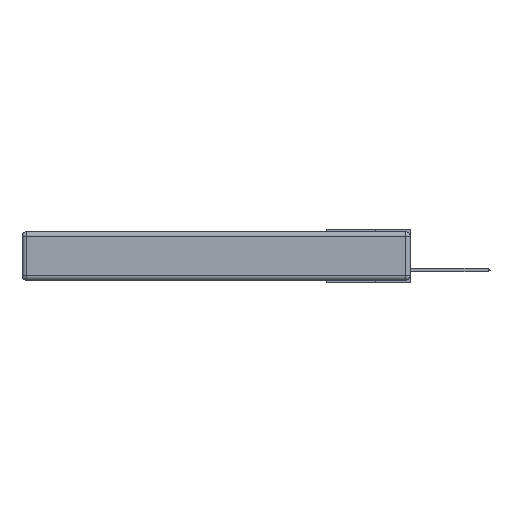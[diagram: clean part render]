
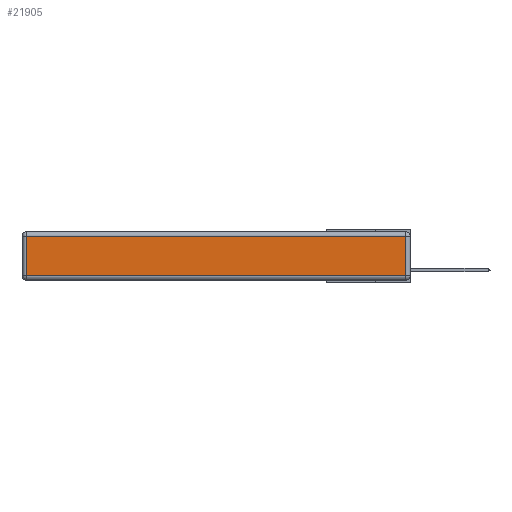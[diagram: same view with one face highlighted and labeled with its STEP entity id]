
A CAD part, left-side view. The second image highlights one B-rep face of the part: STEP entity #21905.
In plain terms, the highlighted planar face has unit normal (-1, 0, 0).
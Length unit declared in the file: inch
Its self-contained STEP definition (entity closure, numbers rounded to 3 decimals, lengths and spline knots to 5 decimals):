
#829 = VECTOR ( 'NONE', #23057, 39.37008 ) ;
#1310 = CARTESIAN_POINT ( 'NONE',  ( 0., 2.72, -0.343 ) ) ;
#1748 = ORIENTED_EDGE ( 'NONE', *, *, #15482, .T. ) ;
#3107 = CARTESIAN_POINT ( 'NONE',  ( 0., 2.72, -0.313 ) ) ;
#3405 = DIRECTION ( 'NONE',  ( 0., 0., 1. ) ) ;
#4110 = CARTESIAN_POINT ( 'NONE',  ( 0., 0., -0.343 ) ) ;
#4360 = FACE_OUTER_BOUND ( 'NONE', #23203, .T. ) ;
#4578 = CARTESIAN_POINT ( 'NONE',  ( 0., 2.72, -0.03 ) ) ;
#5504 = CARTESIAN_POINT ( 'NONE',  ( 0., 0.03, -0.03 ) ) ;
#5834 = LINE ( 'NONE', #1310, #16035 ) ;
#6849 = CARTESIAN_POINT ( 'NONE',  ( 0., 0.03, -0.313 ) ) ;
#7500 = ORIENTED_EDGE ( 'NONE', *, *, #12608, .T. ) ;
#8738 = ORIENTED_EDGE ( 'NONE', *, *, #14990, .T. ) ;
#12608 = EDGE_CURVE ( 'NONE', #20358, #20568, #19639, .T. ) ;
#13585 = VERTEX_POINT ( 'NONE', #4578 ) ;
#13968 = CARTESIAN_POINT ( 'NONE',  ( 0., 2.75, -0.03 ) ) ;
#14410 = AXIS2_PLACEMENT_3D ( 'NONE', #4110, #25110, #3405 ) ;
#14946 = ORIENTED_EDGE ( 'NONE', *, *, #26961, .T. ) ;
#14990 = EDGE_CURVE ( 'NONE', #20568, #25795, #22306, .T. ) ;
#15066 = DIRECTION ( 'NONE',  ( 0., 0., -1. ) ) ;
#15209 = DIRECTION ( 'NONE',  ( 0., -1., 0. ) ) ;
#15482 = EDGE_CURVE ( 'NONE', #25795, #13585, #22269, .T. ) ;
#16035 = VECTOR ( 'NONE', #15066, 39.37008 ) ;
#19605 = CARTESIAN_POINT ( 'NONE',  ( 0., 0., -0.313 ) ) ;
#19639 = LINE ( 'NONE', #19605, #27043 ) ;
#20358 = VERTEX_POINT ( 'NONE', #3107 ) ;
#20568 = VERTEX_POINT ( 'NONE', #6849 ) ;
#21048 = CARTESIAN_POINT ( 'NONE',  ( 0., 0.03, -0.343 ) ) ;
#21905 = ADVANCED_FACE ( 'NONE', ( #4360 ), #24318, .T. ) ;
#22269 = LINE ( 'NONE', #13968, #829 ) ;
#22306 = LINE ( 'NONE', #21048, #24755 ) ;
#23057 = DIRECTION ( 'NONE',  ( 0., 1., 0. ) ) ;
#23203 = EDGE_LOOP ( 'NONE', ( #7500, #8738, #1748, #14946 ) ) ;
#24318 = PLANE ( 'NONE',  #14410 ) ;
#24755 = VECTOR ( 'NONE', #27819, 39.37008 ) ;
#25110 = DIRECTION ( 'NONE',  ( -1., 0., 0. ) ) ;
#25795 = VERTEX_POINT ( 'NONE', #5504 ) ;
#26961 = EDGE_CURVE ( 'NONE', #13585, #20358, #5834, .T. ) ;
#27043 = VECTOR ( 'NONE', #15209, 39.37008 ) ;
#27819 = DIRECTION ( 'NONE',  ( 0., 0., 1. ) ) ;
